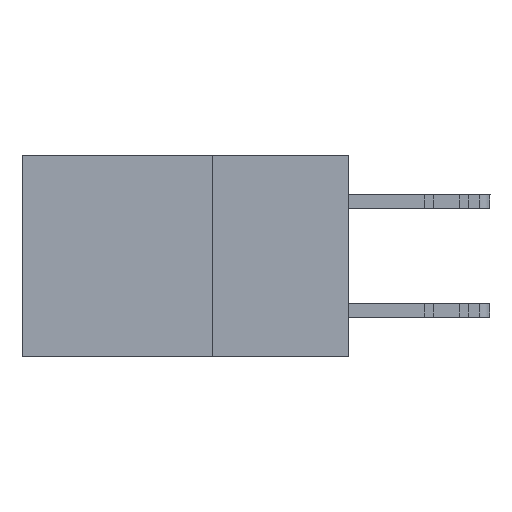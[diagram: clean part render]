
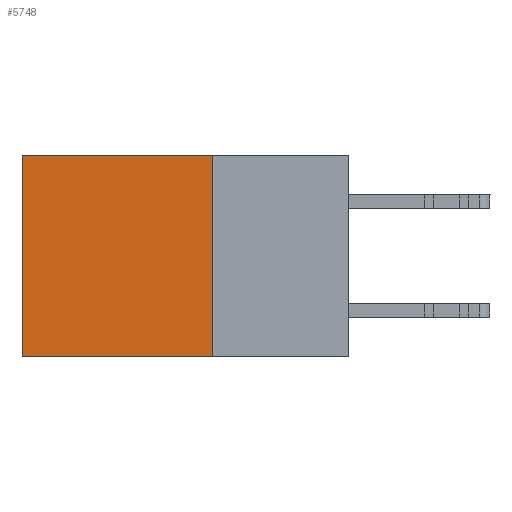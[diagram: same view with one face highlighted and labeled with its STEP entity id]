
A CAD part, left-side view. The second image highlights one B-rep face of the part: STEP entity #5748.
In plain terms, the highlighted planar face has unit normal (-1, 0, 0).
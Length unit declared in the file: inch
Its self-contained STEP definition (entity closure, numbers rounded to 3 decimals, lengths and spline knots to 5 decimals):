
#1088 = CARTESIAN_POINT ( 'NONE',  ( 0.298, 0.25, -0.37 ) ) ;
#1578 = EDGE_CURVE ( 'NONE', #16903, #32704, #19885, .T. ) ;
#3008 = VECTOR ( 'NONE', #7815, 39.37008 ) ;
#4054 = DIRECTION ( 'NONE',  ( 0., 1., 0. ) ) ;
#5649 = VECTOR ( 'NONE', #24948, 39.37008 ) ;
#5748 = ADVANCED_FACE ( 'NONE', ( #31946 ), #26561, .F. ) ;
#5986 = VECTOR ( 'NONE', #4054, 39.37008 ) ;
#6122 = CARTESIAN_POINT ( 'NONE',  ( 0.298, 0.25, 0. ) ) ;
#6465 = DIRECTION ( 'NONE',  ( 1., 0., 0. ) ) ;
#7815 = DIRECTION ( 'NONE',  ( 0., 1., 0. ) ) ;
#9121 = ORIENTED_EDGE ( 'NONE', *, *, #23985, .F. ) ;
#9707 = LINE ( 'NONE', #29798, #5649 ) ;
#10184 = ORIENTED_EDGE ( 'NONE', *, *, #14106, .T. ) ;
#11797 = CARTESIAN_POINT ( 'NONE',  ( 0.298, 0.25, -0.37 ) ) ;
#13372 = CARTESIAN_POINT ( 'NONE',  ( 0.298, 0.6, -0.37 ) ) ;
#13883 = VERTEX_POINT ( 'NONE', #13372 ) ;
#14106 = EDGE_CURVE ( 'NONE', #32704, #13883, #9707, .T. ) ;
#16903 = VERTEX_POINT ( 'NONE', #28198 ) ;
#17272 = ORIENTED_EDGE ( 'NONE', *, *, #1578, .T. ) ;
#18464 = LINE ( 'NONE', #23684, #19879 ) ;
#18964 = DIRECTION ( 'NONE',  ( 0., 0., -1. ) ) ;
#19023 = DIRECTION ( 'NONE',  ( 0., 0., -1. ) ) ;
#19879 = VECTOR ( 'NONE', #18964, 39.37008 ) ;
#19885 = LINE ( 'NONE', #22581, #3008 ) ;
#21524 = AXIS2_PLACEMENT_3D ( 'NONE', #6122, #6465, #19023 ) ;
#21777 = VERTEX_POINT ( 'NONE', #1088 ) ;
#22581 = CARTESIAN_POINT ( 'NONE',  ( 0.298, 0.25, 0. ) ) ;
#23684 = CARTESIAN_POINT ( 'NONE',  ( 0.298, 0.25, 0. ) ) ;
#23985 = EDGE_CURVE ( 'NONE', #16903, #21777, #18464, .T. ) ;
#24516 = EDGE_CURVE ( 'NONE', #21777, #13883, #27058, .T. ) ;
#24948 = DIRECTION ( 'NONE',  ( 0., 0., -1. ) ) ;
#26561 = PLANE ( 'NONE',  #21524 ) ;
#27058 = LINE ( 'NONE', #11797, #5986 ) ;
#28198 = CARTESIAN_POINT ( 'NONE',  ( 0.298, 0.25, 0. ) ) ;
#28836 = ORIENTED_EDGE ( 'NONE', *, *, #24516, .F. ) ;
#29798 = CARTESIAN_POINT ( 'NONE',  ( 0.298, 0.6, 0. ) ) ;
#31688 = EDGE_LOOP ( 'NONE', ( #10184, #28836, #9121, #17272 ) ) ;
#31946 = FACE_OUTER_BOUND ( 'NONE', #31688, .T. ) ;
#32275 = CARTESIAN_POINT ( 'NONE',  ( 0.298, 0.6, 0. ) ) ;
#32704 = VERTEX_POINT ( 'NONE', #32275 ) ;
